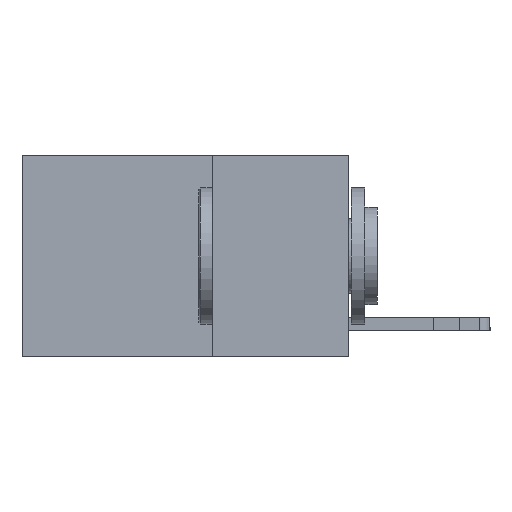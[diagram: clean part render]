
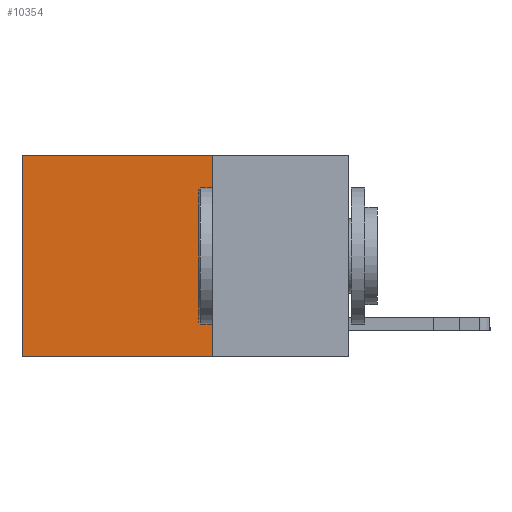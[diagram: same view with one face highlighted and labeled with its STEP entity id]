
A CAD part, left-side view. The second image highlights one B-rep face of the part: STEP entity #10354.
In plain terms, the highlighted planar face has unit normal (-1, 0, 0).
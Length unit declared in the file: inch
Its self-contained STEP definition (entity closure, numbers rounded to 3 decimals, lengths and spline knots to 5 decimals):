
#223 = VERTEX_POINT ( 'NONE', #782 ) ;
#353 = LINE ( 'NONE', #3253, #12148 ) ;
#492 = VECTOR ( 'NONE', #4398, 39.37008 ) ;
#782 = CARTESIAN_POINT ( 'NONE',  ( 0.2625, 0.25, -0.37 ) ) ;
#1251 = PLANE ( 'NONE',  #11240 ) ;
#1456 = CARTESIAN_POINT ( 'NONE',  ( 0.2625, 0.6, -0.37 ) ) ;
#1483 = LINE ( 'NONE', #6311, #492 ) ;
#2390 = DIRECTION ( 'NONE',  ( 0., 1., 0. ) ) ;
#3253 = CARTESIAN_POINT ( 'NONE',  ( 0.2625, 0.25, 0. ) ) ;
#3491 = DIRECTION ( 'NONE',  ( 1., 0., 0. ) ) ;
#3856 = CARTESIAN_POINT ( 'NONE',  ( 0.2625, 0.25, 0. ) ) ;
#4031 = VECTOR ( 'NONE', #6762, 39.37008 ) ;
#4229 = CARTESIAN_POINT ( 'NONE',  ( 0.2625, 0.25, -0.37 ) ) ;
#4355 = EDGE_CURVE ( 'NONE', #10726, #223, #353, .T. ) ;
#4398 = DIRECTION ( 'NONE',  ( 0., 0., -1. ) ) ;
#4614 = ORIENTED_EDGE ( 'NONE', *, *, #4355, .F. ) ;
#5359 = DIRECTION ( 'NONE',  ( 0., 0., -1. ) ) ;
#5518 = ORIENTED_EDGE ( 'NONE', *, *, #9931, .F. ) ;
#5886 = EDGE_LOOP ( 'NONE', ( #12785, #5518, #4614, #12125 ) ) ;
#6311 = CARTESIAN_POINT ( 'NONE',  ( 0.2625, 0.6, 0. ) ) ;
#6612 = VERTEX_POINT ( 'NONE', #10229 ) ;
#6762 = DIRECTION ( 'NONE',  ( 0., 1., 0. ) ) ;
#7511 = DIRECTION ( 'NONE',  ( 0., 0., -1. ) ) ;
#7710 = EDGE_CURVE ( 'NONE', #6612, #8596, #1483, .T. ) ;
#8513 = FACE_OUTER_BOUND ( 'NONE', #5886, .T. ) ;
#8596 = VERTEX_POINT ( 'NONE', #1456 ) ;
#9118 = EDGE_CURVE ( 'NONE', #10726, #6612, #11792, .T. ) ;
#9431 = CARTESIAN_POINT ( 'NONE',  ( 0.2625, 0.25, 0. ) ) ;
#9931 = EDGE_CURVE ( 'NONE', #223, #8596, #10570, .T. ) ;
#10229 = CARTESIAN_POINT ( 'NONE',  ( 0.2625, 0.6, 0. ) ) ;
#10354 = ADVANCED_FACE ( 'NONE', ( #8513 ), #1251, .F. ) ;
#10391 = VECTOR ( 'NONE', #2390, 39.37008 ) ;
#10570 = LINE ( 'NONE', #4229, #10391 ) ;
#10726 = VERTEX_POINT ( 'NONE', #9431 ) ;
#11240 = AXIS2_PLACEMENT_3D ( 'NONE', #12553, #3491, #7511 ) ;
#11792 = LINE ( 'NONE', #3856, #4031 ) ;
#12125 = ORIENTED_EDGE ( 'NONE', *, *, #9118, .T. ) ;
#12148 = VECTOR ( 'NONE', #5359, 39.37008 ) ;
#12553 = CARTESIAN_POINT ( 'NONE',  ( 0.2625, 0.25, 0. ) ) ;
#12785 = ORIENTED_EDGE ( 'NONE', *, *, #7710, .T. ) ;
